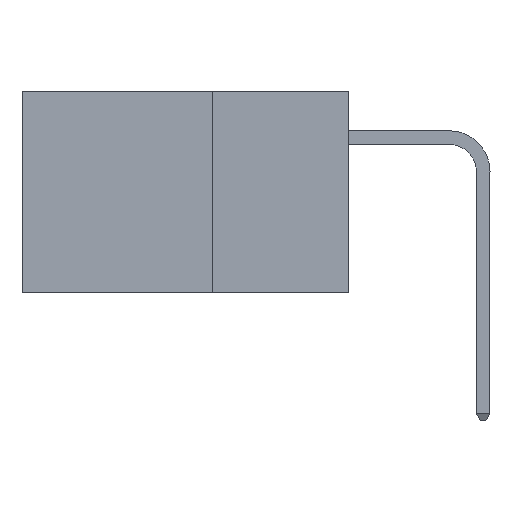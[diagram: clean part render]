
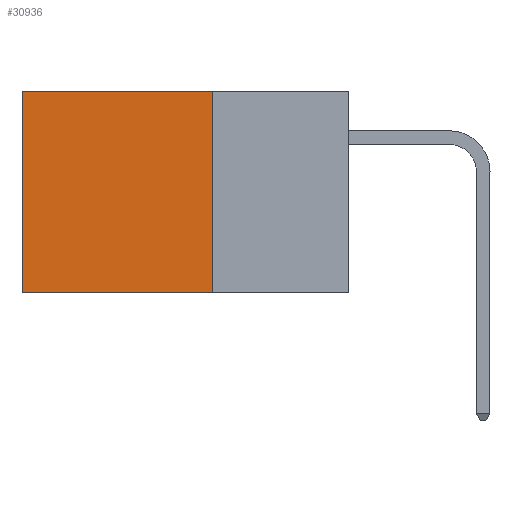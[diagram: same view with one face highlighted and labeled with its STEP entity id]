
A CAD part, left-side view. The second image highlights one B-rep face of the part: STEP entity #30936.
In plain terms, the highlighted planar face has unit normal (-1, 0, 0).
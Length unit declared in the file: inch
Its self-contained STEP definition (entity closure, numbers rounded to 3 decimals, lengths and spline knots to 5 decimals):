
#761 = CARTESIAN_POINT ( 'NONE',  ( 0.2875, 0.25, 0. ) ) ;
#1201 = CARTESIAN_POINT ( 'NONE',  ( 0.2875, 0.25, -0.37 ) ) ;
#1877 = LINE ( 'NONE', #19439, #31614 ) ;
#3105 = DIRECTION ( 'NONE',  ( 0., 0., -1. ) ) ;
#3643 = DIRECTION ( 'NONE',  ( 0., 0., -1. ) ) ;
#4183 = DIRECTION ( 'NONE',  ( 0., 1., 0. ) ) ;
#4258 = CARTESIAN_POINT ( 'NONE',  ( 0.2875, 0.6, 0. ) ) ;
#5307 = CARTESIAN_POINT ( 'NONE',  ( 0.2875, 0.25, -0.37 ) ) ;
#6080 = CARTESIAN_POINT ( 'NONE',  ( 0.2875, 0.6, 0. ) ) ;
#6131 = CARTESIAN_POINT ( 'NONE',  ( 0.2875, 0.25, 0. ) ) ;
#6764 = EDGE_CURVE ( 'NONE', #12198, #12031, #26046, .T. ) ;
#7492 = ORIENTED_EDGE ( 'NONE', *, *, #23329, .T. ) ;
#8612 = ORIENTED_EDGE ( 'NONE', *, *, #11419, .T. ) ;
#9225 = EDGE_LOOP ( 'NONE', ( #8612, #18124, #19033, #7492 ) ) ;
#10042 = VECTOR ( 'NONE', #29108, 39.37008 ) ;
#11419 = EDGE_CURVE ( 'NONE', #18504, #12031, #14240, .T. ) ;
#12031 = VERTEX_POINT ( 'NONE', #16307 ) ;
#12198 = VERTEX_POINT ( 'NONE', #5307 ) ;
#12974 = EDGE_CURVE ( 'NONE', #36859, #12198, #33685, .T. ) ;
#14240 = LINE ( 'NONE', #6080, #36027 ) ;
#14773 = FACE_OUTER_BOUND ( 'NONE', #9225, .T. ) ;
#16307 = CARTESIAN_POINT ( 'NONE',  ( 0.2875, 0.6, -0.37 ) ) ;
#18124 = ORIENTED_EDGE ( 'NONE', *, *, #6764, .F. ) ;
#18166 = CARTESIAN_POINT ( 'NONE',  ( 0.2875, 0.25, 0. ) ) ;
#18486 = VECTOR ( 'NONE', #4183, 39.37008 ) ;
#18504 = VERTEX_POINT ( 'NONE', #4258 ) ;
#19033 = ORIENTED_EDGE ( 'NONE', *, *, #12974, .F. ) ;
#19439 = CARTESIAN_POINT ( 'NONE',  ( 0.2875, 0.25, 0. ) ) ;
#21028 = PLANE ( 'NONE',  #35711 ) ;
#23329 = EDGE_CURVE ( 'NONE', #36859, #18504, #1877, .T. ) ;
#26046 = LINE ( 'NONE', #1201, #18486 ) ;
#29108 = DIRECTION ( 'NONE',  ( 0., 0., -1. ) ) ;
#29495 = DIRECTION ( 'NONE',  ( 1., 0., 0. ) ) ;
#30874 = DIRECTION ( 'NONE',  ( 0., 1., 0. ) ) ;
#30936 = ADVANCED_FACE ( 'NONE', ( #14773 ), #21028, .F. ) ;
#31614 = VECTOR ( 'NONE', #30874, 39.37008 ) ;
#33685 = LINE ( 'NONE', #6131, #10042 ) ;
#35711 = AXIS2_PLACEMENT_3D ( 'NONE', #18166, #29495, #3643 ) ;
#36027 = VECTOR ( 'NONE', #3105, 39.37008 ) ;
#36859 = VERTEX_POINT ( 'NONE', #761 ) ;
